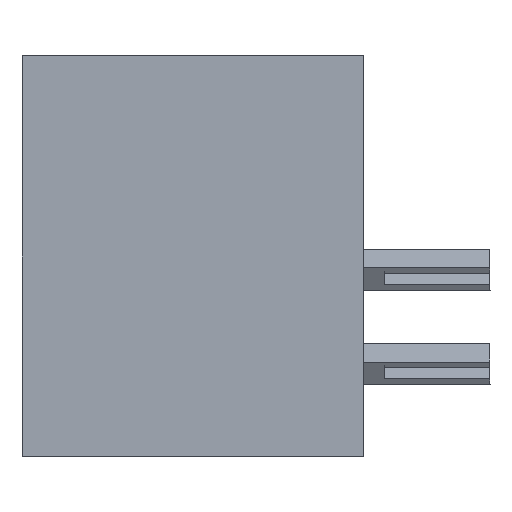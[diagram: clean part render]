
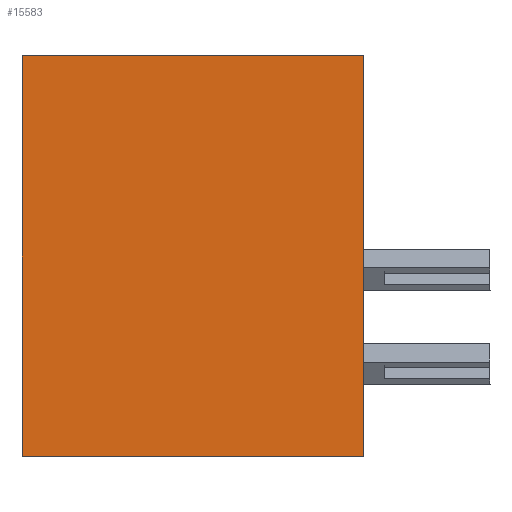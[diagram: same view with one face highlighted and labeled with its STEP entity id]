
A CAD part, left-side view. The second image highlights one B-rep face of the part: STEP entity #15583.
In plain terms, the highlighted planar face has unit normal (-1, 0, 0).
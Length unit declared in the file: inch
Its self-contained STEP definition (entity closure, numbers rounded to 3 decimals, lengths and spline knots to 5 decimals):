
#559 = CARTESIAN_POINT ( 'NONE',  ( 0., 0., -0.531 ) ) ;
#843 = DIRECTION ( 'NONE',  ( 0., 0., 1. ) ) ;
#2106 = LINE ( 'NONE', #5412, #10388 ) ;
#2477 = PLANE ( 'NONE',  #22090 ) ;
#3954 = DIRECTION ( 'NONE',  ( 1., 0., 0. ) ) ;
#4165 = VERTEX_POINT ( 'NONE', #559 ) ;
#5412 = CARTESIAN_POINT ( 'NONE',  ( 0., 0., 0. ) ) ;
#5720 = LINE ( 'NONE', #10555, #10137 ) ;
#6437 = LINE ( 'NONE', #17819, #7801 ) ;
#6766 = DIRECTION ( 'NONE',  ( 0., -1., 0. ) ) ;
#7043 = VERTEX_POINT ( 'NONE', #14572 ) ;
#7692 = VERTEX_POINT ( 'NONE', #17565 ) ;
#7801 = VECTOR ( 'NONE', #8991, 39.37008 ) ;
#8991 = DIRECTION ( 'NONE',  ( 0., -1., 0. ) ) ;
#10137 = VECTOR ( 'NONE', #6766, 39.37008 ) ;
#10388 = VECTOR ( 'NONE', #21356, 39.37008 ) ;
#10555 = CARTESIAN_POINT ( 'NONE',  ( 0., 0.453, 0. ) ) ;
#10935 = ORIENTED_EDGE ( 'NONE', *, *, #21389, .F. ) ;
#11125 = EDGE_CURVE ( 'NONE', #4165, #7692, #2106, .T. ) ;
#11149 = ORIENTED_EDGE ( 'NONE', *, *, #11125, .T. ) ;
#11192 = ORIENTED_EDGE ( 'NONE', *, *, #15962, .T. ) ;
#12053 = LINE ( 'NONE', #16644, #13698 ) ;
#13217 = VERTEX_POINT ( 'NONE', #18134 ) ;
#13698 = VECTOR ( 'NONE', #843, 39.37008 ) ;
#14572 = CARTESIAN_POINT ( 'NONE',  ( 0., 0.453, -0.531 ) ) ;
#15178 = EDGE_LOOP ( 'NONE', ( #11149, #10935, #21707, #11192 ) ) ;
#15583 = ADVANCED_FACE ( 'NONE', ( #17337 ), #2477, .F. ) ;
#15962 = EDGE_CURVE ( 'NONE', #7043, #4165, #6437, .T. ) ;
#16146 = EDGE_CURVE ( 'NONE', #7043, #13217, #12053, .T. ) ;
#16425 = CARTESIAN_POINT ( 'NONE',  ( 0., 0.453, 0. ) ) ;
#16644 = CARTESIAN_POINT ( 'NONE',  ( 0., 0.453, 0. ) ) ;
#17337 = FACE_OUTER_BOUND ( 'NONE', #15178, .T. ) ;
#17565 = CARTESIAN_POINT ( 'NONE',  ( 0., 0., 0. ) ) ;
#17819 = CARTESIAN_POINT ( 'NONE',  ( 0., 0.453, -0.531 ) ) ;
#18134 = CARTESIAN_POINT ( 'NONE',  ( 0., 0.453, 0. ) ) ;
#19900 = DIRECTION ( 'NONE',  ( 0., 0., -1. ) ) ;
#21356 = DIRECTION ( 'NONE',  ( 0., 0., 1. ) ) ;
#21389 = EDGE_CURVE ( 'NONE', #13217, #7692, #5720, .T. ) ;
#21707 = ORIENTED_EDGE ( 'NONE', *, *, #16146, .F. ) ;
#22090 = AXIS2_PLACEMENT_3D ( 'NONE', #16425, #3954, #19900 ) ;
